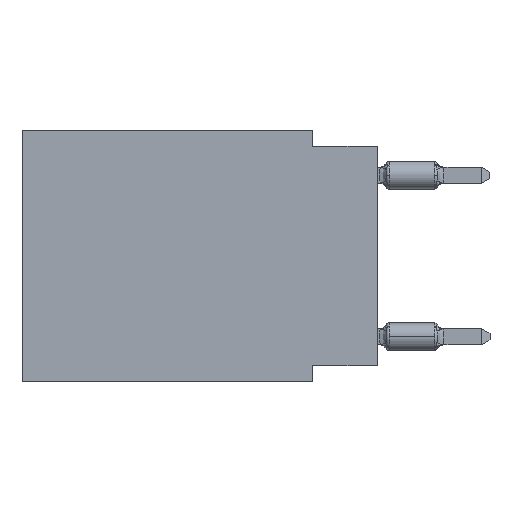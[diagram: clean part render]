
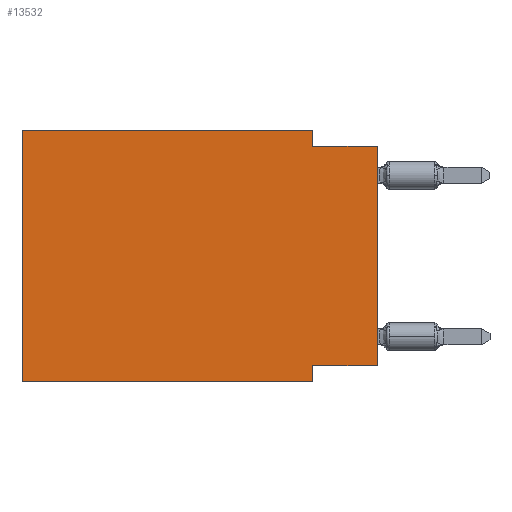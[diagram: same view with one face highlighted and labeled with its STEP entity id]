
A CAD part, left-side view. The second image highlights one B-rep face of the part: STEP entity #13532.
In plain terms, the highlighted planar face has unit normal (-1, 0, 0).
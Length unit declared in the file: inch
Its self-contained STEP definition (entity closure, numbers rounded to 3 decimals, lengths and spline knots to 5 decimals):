
#37 = FACE_OUTER_BOUND ( 'NONE', #245, .T. ) ;
#245 = EDGE_LOOP ( 'NONE', ( #10636, #15162, #5435, #8324, #11016, #2410, #3241, #15720 ) ) ;
#311 = DIRECTION ( 'NONE',  ( 0., -1., 0. ) ) ;
#424 = CARTESIAN_POINT ( 'NONE',  ( 0., 0.1, -0.025 ) ) ;
#560 = CARTESIAN_POINT ( 'NONE',  ( 0., 0.1, 0. ) ) ;
#953 = VERTEX_POINT ( 'NONE', #560 ) ;
#1026 = VECTOR ( 'NONE', #3948, 39.37008 ) ;
#1056 = EDGE_CURVE ( 'NONE', #953, #10562, #4398, .T. ) ;
#1224 = DIRECTION ( 'NONE',  ( 0., 0., -1. ) ) ;
#1589 = CARTESIAN_POINT ( 'NONE',  ( 0., 0.55, 0. ) ) ;
#1629 = LINE ( 'NONE', #10142, #1026 ) ;
#1812 = CARTESIAN_POINT ( 'NONE',  ( 0., 0., -0.365 ) ) ;
#1915 = DIRECTION ( 'NONE',  ( 0., 0., -1. ) ) ;
#2151 = EDGE_CURVE ( 'NONE', #10777, #7605, #1629, .T. ) ;
#2410 = ORIENTED_EDGE ( 'NONE', *, *, #11282, .T. ) ;
#2425 = VERTEX_POINT ( 'NONE', #5823 ) ;
#2589 = CARTESIAN_POINT ( 'NONE',  ( 0., 0., 0. ) ) ;
#2739 = VERTEX_POINT ( 'NONE', #14279 ) ;
#2950 = VECTOR ( 'NONE', #1915, 39.37008 ) ;
#2957 = LINE ( 'NONE', #13642, #14895 ) ;
#3241 = ORIENTED_EDGE ( 'NONE', *, *, #7888, .F. ) ;
#3503 = CARTESIAN_POINT ( 'NONE',  ( 0., 0.55, -0.39 ) ) ;
#3948 = DIRECTION ( 'NONE',  ( 0., 0., 1. ) ) ;
#4133 = EDGE_CURVE ( 'NONE', #7605, #953, #7571, .T. ) ;
#4398 = LINE ( 'NONE', #8932, #11450 ) ;
#5365 = EDGE_CURVE ( 'NONE', #10562, #7158, #2957, .T. ) ;
#5435 = ORIENTED_EDGE ( 'NONE', *, *, #1056, .F. ) ;
#5823 = CARTESIAN_POINT ( 'NONE',  ( 0., 0.1, -0.39 ) ) ;
#6136 = CARTESIAN_POINT ( 'NONE',  ( 0., 0.55, -0.39 ) ) ;
#6203 = DIRECTION ( 'NONE',  ( 0., -1., 0. ) ) ;
#7158 = VERTEX_POINT ( 'NONE', #13427 ) ;
#7169 = EDGE_CURVE ( 'NONE', #11424, #7158, #7358, .T. ) ;
#7358 = LINE ( 'NONE', #2589, #13243 ) ;
#7571 = LINE ( 'NONE', #1589, #8719 ) ;
#7605 = VERTEX_POINT ( 'NONE', #12044 ) ;
#7888 = EDGE_CURVE ( 'NONE', #2739, #2425, #9001, .T. ) ;
#8324 = ORIENTED_EDGE ( 'NONE', *, *, #4133, .F. ) ;
#8719 = VECTOR ( 'NONE', #12270, 39.37008 ) ;
#8932 = CARTESIAN_POINT ( 'NONE',  ( 0., 0.1, 0. ) ) ;
#9001 = LINE ( 'NONE', #13890, #2950 ) ;
#9204 = VECTOR ( 'NONE', #9982, 39.37008 ) ;
#9419 = AXIS2_PLACEMENT_3D ( 'NONE', #9681, #14725, #1224 ) ;
#9681 = CARTESIAN_POINT ( 'NONE',  ( 0., 0.55, 0. ) ) ;
#9982 = DIRECTION ( 'NONE',  ( 0., 1., 0. ) ) ;
#10142 = CARTESIAN_POINT ( 'NONE',  ( 0., 0.55, 0. ) ) ;
#10562 = VERTEX_POINT ( 'NONE', #424 ) ;
#10636 = ORIENTED_EDGE ( 'NONE', *, *, #7169, .T. ) ;
#10760 = DIRECTION ( 'NONE',  ( 0., 0., -1. ) ) ;
#10777 = VERTEX_POINT ( 'NONE', #6136 ) ;
#11016 = ORIENTED_EDGE ( 'NONE', *, *, #2151, .F. ) ;
#11118 = LINE ( 'NONE', #15740, #9204 ) ;
#11206 = PLANE ( 'NONE',  #9419 ) ;
#11282 = EDGE_CURVE ( 'NONE', #10777, #2425, #13387, .T. ) ;
#11424 = VERTEX_POINT ( 'NONE', #1812 ) ;
#11450 = VECTOR ( 'NONE', #10760, 39.37008 ) ;
#12044 = CARTESIAN_POINT ( 'NONE',  ( 0., 0.55, 0. ) ) ;
#12215 = DIRECTION ( 'NONE',  ( 0., 0., 1. ) ) ;
#12270 = DIRECTION ( 'NONE',  ( 0., -1., 0. ) ) ;
#13243 = VECTOR ( 'NONE', #12215, 39.37008 ) ;
#13387 = LINE ( 'NONE', #3503, #14668 ) ;
#13427 = CARTESIAN_POINT ( 'NONE',  ( 0., 0., -0.025 ) ) ;
#13532 = ADVANCED_FACE ( 'NONE', ( #37 ), #11206, .F. ) ;
#13642 = CARTESIAN_POINT ( 'NONE',  ( 0., 0., -0.025 ) ) ;
#13890 = CARTESIAN_POINT ( 'NONE',  ( 0., 0.1, -0.39 ) ) ;
#14279 = CARTESIAN_POINT ( 'NONE',  ( 0., 0.1, -0.365 ) ) ;
#14668 = VECTOR ( 'NONE', #6203, 39.37008 ) ;
#14725 = DIRECTION ( 'NONE',  ( 1., 0., 0. ) ) ;
#14895 = VECTOR ( 'NONE', #311, 39.37008 ) ;
#15162 = ORIENTED_EDGE ( 'NONE', *, *, #5365, .F. ) ;
#15201 = EDGE_CURVE ( 'NONE', #11424, #2739, #11118, .T. ) ;
#15720 = ORIENTED_EDGE ( 'NONE', *, *, #15201, .F. ) ;
#15740 = CARTESIAN_POINT ( 'NONE',  ( 0., 0., -0.365 ) ) ;
